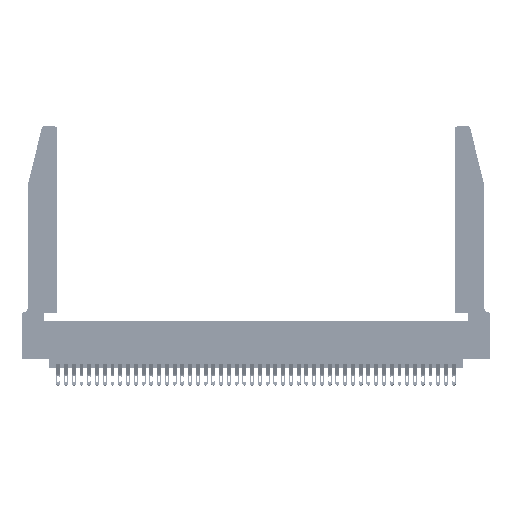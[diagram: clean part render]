
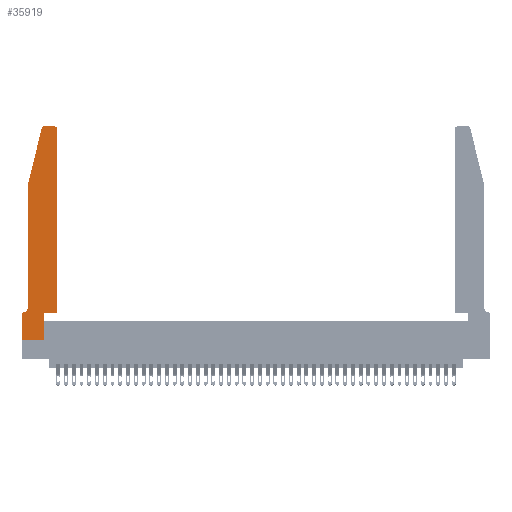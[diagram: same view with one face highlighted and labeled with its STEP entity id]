
A CAD part, top view. The second image highlights one B-rep face of the part: STEP entity #35919.
In plain terms, the highlighted planar face has unit normal (0, 0, 1).
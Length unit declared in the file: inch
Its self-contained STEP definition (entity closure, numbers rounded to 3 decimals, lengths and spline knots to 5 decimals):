
#183 = PLANE ( 'NONE',  #8959 ) ;
#342 = EDGE_CURVE ( 'NONE', #18371, #2012, #29690, .T. ) ;
#505 = EDGE_LOOP ( 'NONE', ( #11070, #36117, #44203, #10682, #38341, #22256, #18688, #26403, #43843, #34054, #13120, #28202 ) ) ;
#1000 = DIRECTION ( 'NONE',  ( -1., 0., 0. ) ) ;
#1983 = EDGE_CURVE ( 'NONE', #36315, #18371, #30126, .T. ) ;
#2012 = VERTEX_POINT ( 'NONE', #39224 ) ;
#2069 = CARTESIAN_POINT ( 'NONE',  ( 0.0755, 2., 0.37 ) ) ;
#3086 = CARTESIAN_POINT ( 'NONE',  ( 0.0755, 0.35, 0.37 ) ) ;
#3150 = EDGE_CURVE ( 'NONE', #42979, #36315, #35525, .T. ) ;
#3578 = CARTESIAN_POINT ( 'NONE',  ( 0.4205, 2.72, 0.37 ) ) ;
#4236 = CARTESIAN_POINT ( 'NONE',  ( 0., 0., 0.37 ) ) ;
#7229 = DIRECTION ( 'NONE',  ( -1., 0., 0. ) ) ;
#8536 = VECTOR ( 'NONE', #12311, 39.37008 ) ;
#8959 = AXIS2_PLACEMENT_3D ( 'NONE', #31607, #41978, #17968 ) ;
#9952 = CARTESIAN_POINT ( 'NONE',  ( 0.0755, 2., 0.37 ) ) ;
#9970 = VERTEX_POINT ( 'NONE', #22575 ) ;
#10060 = DIRECTION ( 'NONE',  ( 1., 0., 0. ) ) ;
#10364 = EDGE_CURVE ( 'NONE', #20773, #36245, #29172, .T. ) ;
#10529 = DIRECTION ( 'NONE',  ( 0., 1., 0. ) ) ;
#10628 = CARTESIAN_POINT ( 'NONE',  ( 0., 0., 0.37 ) ) ;
#10682 = ORIENTED_EDGE ( 'NONE', *, *, #34370, .T. ) ;
#11070 = ORIENTED_EDGE ( 'NONE', *, *, #24629, .T. ) ;
#11249 = LINE ( 'NONE', #10628, #15128 ) ;
#11414 = CARTESIAN_POINT ( 'NONE',  ( 0.284, 2.75, 0.37 ) ) ;
#11590 = CARTESIAN_POINT ( 'NONE',  ( 0.0055, 0.42, 0.37 ) ) ;
#11872 = CARTESIAN_POINT ( 'NONE',  ( 0.2865, 0., 0.37 ) ) ;
#12026 = VECTOR ( 'NONE', #1000, 39.37008 ) ;
#12311 = DIRECTION ( 'NONE',  ( 0., -1., 0. ) ) ;
#13009 = CIRCLE ( 'NONE', #16373, 0.07 ) ;
#13120 = ORIENTED_EDGE ( 'NONE', *, *, #35900, .T. ) ;
#13411 = EDGE_CURVE ( 'NONE', #28929, #39931, #31028, .T. ) ;
#15128 = VECTOR ( 'NONE', #24305, 39.37008 ) ;
#15561 = EDGE_CURVE ( 'NONE', #9970, #20773, #13009, .T. ) ;
#16084 = VECTOR ( 'NONE', #28330, 39.37008 ) ;
#16185 = AXIS2_PLACEMENT_3D ( 'NONE', #3578, #31163, #27839 ) ;
#16373 = AXIS2_PLACEMENT_3D ( 'NONE', #11590, #40950, #7229 ) ;
#16699 = VECTOR ( 'NONE', #24860, 39.37008 ) ;
#17728 = VERTEX_POINT ( 'NONE', #9952 ) ;
#17968 = DIRECTION ( 'NONE',  ( 1., 0., 0. ) ) ;
#18371 = VERTEX_POINT ( 'NONE', #19007 ) ;
#18420 = VERTEX_POINT ( 'NONE', #20381 ) ;
#18688 = ORIENTED_EDGE ( 'NONE', *, *, #38723, .T. ) ;
#19007 = CARTESIAN_POINT ( 'NONE',  ( 0.2865, 0.35, 0.37 ) ) ;
#20381 = CARTESIAN_POINT ( 'NONE',  ( 0.4205, 2.75, 0.37 ) ) ;
#20773 = VERTEX_POINT ( 'NONE', #37250 ) ;
#21244 = LINE ( 'NONE', #38962, #12026 ) ;
#21813 = FACE_OUTER_BOUND ( 'NONE', #505, .T. ) ;
#22136 = CARTESIAN_POINT ( 'NONE',  ( 0.0755, 2., 0.37 ) ) ;
#22256 = ORIENTED_EDGE ( 'NONE', *, *, #10364, .T. ) ;
#22575 = CARTESIAN_POINT ( 'NONE',  ( 0.0755, 0.42, 0.37 ) ) ;
#24305 = DIRECTION ( 'NONE',  ( 0., -1., 0. ) ) ;
#24431 = CARTESIAN_POINT ( 'NONE',  ( 0.25487, 2.72718, 0.37 ) ) ;
#24594 = LINE ( 'NONE', #22136, #43511 ) ;
#24629 = EDGE_CURVE ( 'NONE', #18420, #28929, #21244, .T. ) ;
#24860 = DIRECTION ( 'NONE',  ( -1., 0., 0. ) ) ;
#24992 = DIRECTION ( 'NONE',  ( 0., 1., 0. ) ) ;
#25434 = CARTESIAN_POINT ( 'NONE',  ( 0.4505, 2.72, 0.37 ) ) ;
#26017 = DIRECTION ( 'NONE',  ( 0., 0., 1. ) ) ;
#26403 = ORIENTED_EDGE ( 'NONE', *, *, #3150, .T. ) ;
#27513 = VECTOR ( 'NONE', #10060, 39.37008 ) ;
#27839 = DIRECTION ( 'NONE',  ( 1., 0., 0. ) ) ;
#27844 = CARTESIAN_POINT ( 'NONE',  ( 0.4505, 0.35, 0.37 ) ) ;
#28202 = ORIENTED_EDGE ( 'NONE', *, *, #32802, .T. ) ;
#28239 = CIRCLE ( 'NONE', #16185, 0.03 ) ;
#28330 = DIRECTION ( 'NONE',  ( 1., 0., 0. ) ) ;
#28795 = CARTESIAN_POINT ( 'NONE',  ( 0.2865, 0.35, 0.37 ) ) ;
#28929 = VERTEX_POINT ( 'NONE', #11414 ) ;
#29172 = LINE ( 'NONE', #3086, #16699 ) ;
#29657 = DIRECTION ( 'NONE',  ( 1., 0., 0. ) ) ;
#29690 = LINE ( 'NONE', #30802, #27513 ) ;
#30126 = LINE ( 'NONE', #28795, #34936 ) ;
#30802 = CARTESIAN_POINT ( 'NONE',  ( 0.4505, 0.35, 0.37 ) ) ;
#31028 = CIRCLE ( 'NONE', #36579, 0.03 ) ;
#31163 = DIRECTION ( 'NONE',  ( 0., 0., 1. ) ) ;
#31607 = CARTESIAN_POINT ( 'NONE',  ( 0., 0.35, 0.37 ) ) ;
#32454 = VERTEX_POINT ( 'NONE', #25434 ) ;
#32626 = LINE ( 'NONE', #27844, #39106 ) ;
#32802 = EDGE_CURVE ( 'NONE', #32454, #18420, #28239, .T. ) ;
#33247 = CARTESIAN_POINT ( 'NONE',  ( 0., 0.35, 0.37 ) ) ;
#33401 = CARTESIAN_POINT ( 'NONE',  ( 0.284, 2.72, 0.37 ) ) ;
#34054 = ORIENTED_EDGE ( 'NONE', *, *, #342, .T. ) ;
#34370 = EDGE_CURVE ( 'NONE', #17728, #9970, #39976, .T. ) ;
#34936 = VECTOR ( 'NONE', #24992, 39.37008 ) ;
#35525 = LINE ( 'NONE', #4236, #16084 ) ;
#35900 = EDGE_CURVE ( 'NONE', #2012, #32454, #32626, .T. ) ;
#35919 = ADVANCED_FACE ( 'NONE', ( #21813 ), #183, .T. ) ;
#36117 = ORIENTED_EDGE ( 'NONE', *, *, #13411, .T. ) ;
#36119 = CARTESIAN_POINT ( 'NONE',  ( 0., 0., 0.37 ) ) ;
#36245 = VERTEX_POINT ( 'NONE', #33247 ) ;
#36315 = VERTEX_POINT ( 'NONE', #11872 ) ;
#36579 = AXIS2_PLACEMENT_3D ( 'NONE', #33401, #26017, #29657 ) ;
#37250 = CARTESIAN_POINT ( 'NONE',  ( 0.0055, 0.35, 0.37 ) ) ;
#38341 = ORIENTED_EDGE ( 'NONE', *, *, #15561, .T. ) ;
#38723 = EDGE_CURVE ( 'NONE', #36245, #42979, #11249, .T. ) ;
#38962 = CARTESIAN_POINT ( 'NONE',  ( 0.2605, 2.75, 0.37 ) ) ;
#39036 = DIRECTION ( 'NONE',  ( -0.239, -0.971, 0. ) ) ;
#39106 = VECTOR ( 'NONE', #10529, 39.37008 ) ;
#39224 = CARTESIAN_POINT ( 'NONE',  ( 0.4505, 0.35, 0.37 ) ) ;
#39931 = VERTEX_POINT ( 'NONE', #24431 ) ;
#39976 = LINE ( 'NONE', #2069, #8536 ) ;
#40950 = DIRECTION ( 'NONE',  ( 0., 0., -1. ) ) ;
#41522 = EDGE_CURVE ( 'NONE', #39931, #17728, #24594, .T. ) ;
#41978 = DIRECTION ( 'NONE',  ( 0., 0., 1. ) ) ;
#42979 = VERTEX_POINT ( 'NONE', #36119 ) ;
#43511 = VECTOR ( 'NONE', #39036, 39.37008 ) ;
#43843 = ORIENTED_EDGE ( 'NONE', *, *, #1983, .T. ) ;
#44203 = ORIENTED_EDGE ( 'NONE', *, *, #41522, .T. ) ;
